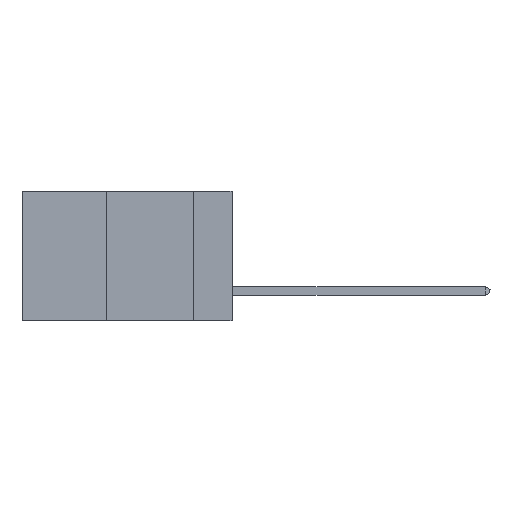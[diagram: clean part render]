
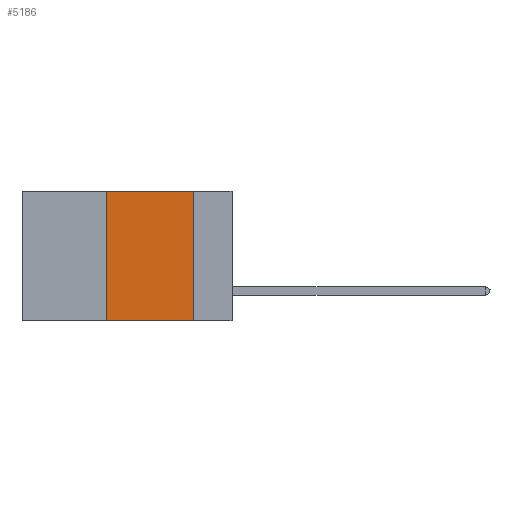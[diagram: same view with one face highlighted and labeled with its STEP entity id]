
A CAD part, left-side view. The second image highlights one B-rep face of the part: STEP entity #5186.
In plain terms, the highlighted planar face has unit normal (-1, 0, 0).
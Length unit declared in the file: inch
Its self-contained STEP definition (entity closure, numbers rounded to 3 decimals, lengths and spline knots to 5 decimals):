
#325 = CARTESIAN_POINT ( 'NONE',  ( 0., 0.36, -0.37 ) ) ;
#1017 = CARTESIAN_POINT ( 'NONE',  ( 0., 0.11, -0.37 ) ) ;
#2250 = VECTOR ( 'NONE', #5221, 39.37008 ) ;
#2284 = VERTEX_POINT ( 'NONE', #325 ) ;
#3449 = EDGE_CURVE ( 'NONE', #14172, #4048, #8208, .T. ) ;
#4048 = VERTEX_POINT ( 'NONE', #1017 ) ;
#4365 = FACE_OUTER_BOUND ( 'NONE', #10727, .T. ) ;
#5074 = LINE ( 'NONE', #12666, #2250 ) ;
#5186 = ADVANCED_FACE ( 'NONE', ( #4365 ), #11157, .F. ) ;
#5221 = DIRECTION ( 'NONE',  ( 0., -1., 0. ) ) ;
#5993 = DIRECTION ( 'NONE',  ( 0., 0., 1. ) ) ;
#6519 = LINE ( 'NONE', #11994, #9563 ) ;
#6916 = ORIENTED_EDGE ( 'NONE', *, *, #3449, .F. ) ;
#7057 = AXIS2_PLACEMENT_3D ( 'NONE', #9699, #18566, #14147 ) ;
#7402 = CARTESIAN_POINT ( 'NONE',  ( 0., 0.36, 0. ) ) ;
#8208 = LINE ( 'NONE', #11832, #8673 ) ;
#8673 = VECTOR ( 'NONE', #12598, 39.37008 ) ;
#8924 = VECTOR ( 'NONE', #5993, 39.37008 ) ;
#9069 = CARTESIAN_POINT ( 'NONE',  ( 0., 0.36, 0. ) ) ;
#9279 = EDGE_CURVE ( 'NONE', #2284, #14326, #17132, .T. ) ;
#9313 = DIRECTION ( 'NONE',  ( 0., -1., 0. ) ) ;
#9563 = VECTOR ( 'NONE', #9313, 39.37008 ) ;
#9699 = CARTESIAN_POINT ( 'NONE',  ( 0., 0.6, 0. ) ) ;
#10727 = EDGE_LOOP ( 'NONE', ( #6916, #11008, #15674, #19404 ) ) ;
#10986 = EDGE_CURVE ( 'NONE', #14326, #14172, #6519, .T. ) ;
#11008 = ORIENTED_EDGE ( 'NONE', *, *, #10986, .F. ) ;
#11157 = PLANE ( 'NONE',  #7057 ) ;
#11832 = CARTESIAN_POINT ( 'NONE',  ( 0., 0.11, 0. ) ) ;
#11994 = CARTESIAN_POINT ( 'NONE',  ( 0., 0.6, 0. ) ) ;
#12598 = DIRECTION ( 'NONE',  ( 0., 0., -1. ) ) ;
#12666 = CARTESIAN_POINT ( 'NONE',  ( 0., 0.6, -0.37 ) ) ;
#14147 = DIRECTION ( 'NONE',  ( 0., 0., -1. ) ) ;
#14172 = VERTEX_POINT ( 'NONE', #17674 ) ;
#14326 = VERTEX_POINT ( 'NONE', #7402 ) ;
#15674 = ORIENTED_EDGE ( 'NONE', *, *, #9279, .F. ) ;
#16225 = EDGE_CURVE ( 'NONE', #2284, #4048, #5074, .T. ) ;
#17132 = LINE ( 'NONE', #9069, #8924 ) ;
#17674 = CARTESIAN_POINT ( 'NONE',  ( 0., 0.11, 0. ) ) ;
#18566 = DIRECTION ( 'NONE',  ( 1., 0., 0. ) ) ;
#19404 = ORIENTED_EDGE ( 'NONE', *, *, #16225, .T. ) ;
